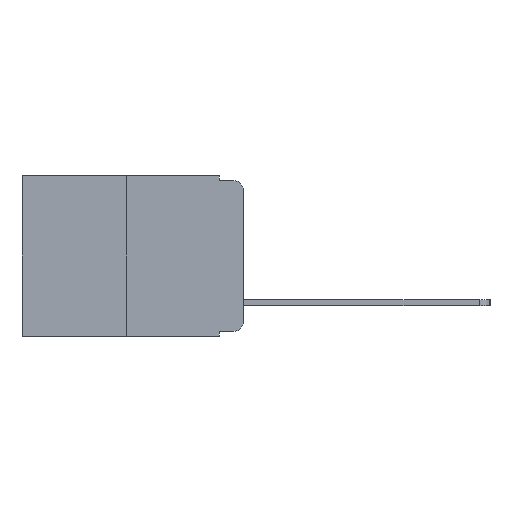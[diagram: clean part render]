
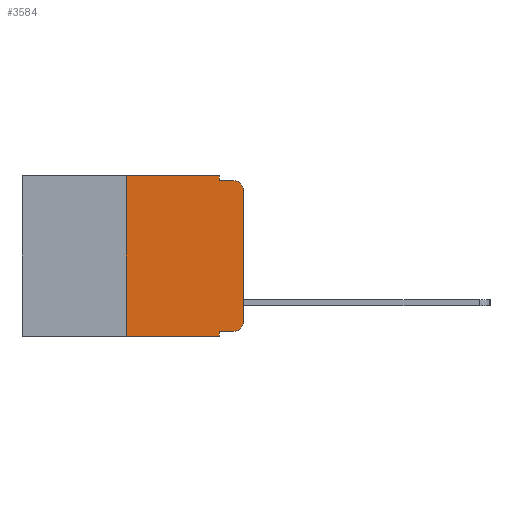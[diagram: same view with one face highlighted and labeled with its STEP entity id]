
A CAD part, left-side view. The second image highlights one B-rep face of the part: STEP entity #3584.
In plain terms, the highlighted planar face has unit normal (-1, 0, 0).
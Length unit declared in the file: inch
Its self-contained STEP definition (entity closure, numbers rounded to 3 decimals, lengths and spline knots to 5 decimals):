
#1 = CARTESIAN_POINT ( 'NONE',  ( 0., 0.25, -0.343 ) ) ;
#11 = EDGE_CURVE ( 'NONE', #4021, #7006, #10398, .T. ) ;
#295 = CARTESIAN_POINT ( 'NONE',  ( 0., 0., 0. ) ) ;
#320 = CARTESIAN_POINT ( 'NONE',  ( 0., 0.051, -0.333 ) ) ;
#432 = EDGE_CURVE ( 'NONE', #691, #3779, #3934, .T. ) ;
#502 = EDGE_CURVE ( 'NONE', #691, #6331, #7375, .T. ) ;
#691 = VERTEX_POINT ( 'NONE', #1 ) ;
#850 = VECTOR ( 'NONE', #9509, 39.37008 ) ;
#1102 = CARTESIAN_POINT ( 'NONE',  ( 0., 0.051, -0.333 ) ) ;
#1162 = VERTEX_POINT ( 'NONE', #320 ) ;
#1263 = CARTESIAN_POINT ( 'NONE',  ( 0., 0.051, -0.01 ) ) ;
#1444 = DIRECTION ( 'NONE',  ( -1., 0., 0. ) ) ;
#1470 = VECTOR ( 'NONE', #6472, 39.37008 ) ;
#1531 = VERTEX_POINT ( 'NONE', #2167 ) ;
#1986 = VECTOR ( 'NONE', #3161, 39.37008 ) ;
#2056 = VERTEX_POINT ( 'NONE', #5298 ) ;
#2109 = VECTOR ( 'NONE', #8835, 39.37008 ) ;
#2159 = LINE ( 'NONE', #10298, #4240 ) ;
#2167 = CARTESIAN_POINT ( 'NONE',  ( 0., 0.051, 0. ) ) ;
#2292 = CARTESIAN_POINT ( 'NONE',  ( 0., 0.25, 0. ) ) ;
#2390 = CARTESIAN_POINT ( 'NONE',  ( 0., 0.051, -0.343 ) ) ;
#2724 = VERTEX_POINT ( 'NONE', #9050 ) ;
#2893 = AXIS2_PLACEMENT_3D ( 'NONE', #6483, #7558, #7539 ) ;
#3161 = DIRECTION ( 'NONE',  ( 0., 0., -1. ) ) ;
#3313 = EDGE_CURVE ( 'NONE', #7006, #8983, #10348, .T. ) ;
#3584 = ADVANCED_FACE ( 'NONE', ( #10341 ), #9592, .F. ) ;
#3779 = VERTEX_POINT ( 'NONE', #2292 ) ;
#3827 = CARTESIAN_POINT ( 'NONE',  ( 0., 0., -0.03 ) ) ;
#3934 = LINE ( 'NONE', #7896, #1470 ) ;
#4021 = VERTEX_POINT ( 'NONE', #8584 ) ;
#4190 = EDGE_CURVE ( 'NONE', #3779, #1531, #2159, .T. ) ;
#4240 = VECTOR ( 'NONE', #8830, 39.37008 ) ;
#4347 = ORIENTED_EDGE ( 'NONE', *, *, #11, .T. ) ;
#4392 = ORIENTED_EDGE ( 'NONE', *, *, #9510, .T. ) ;
#4400 = ORIENTED_EDGE ( 'NONE', *, *, #3313, .T. ) ;
#4497 = EDGE_LOOP ( 'NONE', ( #4347, #4400, #4633, #4656, #8241, #7687, #6742, #6384, #4676, #4392 ) ) ;
#4633 = ORIENTED_EDGE ( 'NONE', *, *, #4934, .F. ) ;
#4656 = ORIENTED_EDGE ( 'NONE', *, *, #8006, .F. ) ;
#4676 = ORIENTED_EDGE ( 'NONE', *, *, #7090, .T. ) ;
#4934 = EDGE_CURVE ( 'NONE', #2724, #8983, #6687, .T. ) ;
#5298 = CARTESIAN_POINT ( 'NONE',  ( 0., 0.02, -0.333 ) ) ;
#5483 = VECTOR ( 'NONE', #9783, 39.37008 ) ;
#5706 = VECTOR ( 'NONE', #9941, 39.37008 ) ;
#5717 = LINE ( 'NONE', #7666, #5483 ) ;
#5943 = DIRECTION ( 'NONE',  ( 0., 0., -1. ) ) ;
#6331 = VERTEX_POINT ( 'NONE', #2390 ) ;
#6347 = CARTESIAN_POINT ( 'NONE',  ( 0., 0.051, 0. ) ) ;
#6384 = ORIENTED_EDGE ( 'NONE', *, *, #6588, .F. ) ;
#6385 = DIRECTION ( 'NONE',  ( -1., 0., 0. ) ) ;
#6472 = DIRECTION ( 'NONE',  ( 0., 0., 1. ) ) ;
#6483 = CARTESIAN_POINT ( 'NONE',  ( 0., 0.473, 0. ) ) ;
#6540 = CARTESIAN_POINT ( 'NONE',  ( 0., 0.02, -0.313 ) ) ;
#6588 = EDGE_CURVE ( 'NONE', #1162, #6331, #5717, .T. ) ;
#6687 = LINE ( 'NONE', #1263, #8615 ) ;
#6696 = LINE ( 'NONE', #6347, #1986 ) ;
#6742 = ORIENTED_EDGE ( 'NONE', *, *, #502, .T. ) ;
#7006 = VERTEX_POINT ( 'NONE', #3827 ) ;
#7090 = EDGE_CURVE ( 'NONE', #1162, #2056, #7758, .T. ) ;
#7177 = DIRECTION ( 'NONE',  ( 0., -1., 0. ) ) ;
#7323 = DIRECTION ( 'NONE',  ( 0., 0., -1. ) ) ;
#7375 = LINE ( 'NONE', #10289, #850 ) ;
#7397 = CIRCLE ( 'NONE', #7849, 0.02 ) ;
#7539 = DIRECTION ( 'NONE',  ( 0., 0., -1. ) ) ;
#7558 = DIRECTION ( 'NONE',  ( 1., 0., 0. ) ) ;
#7666 = CARTESIAN_POINT ( 'NONE',  ( 0., 0.051, 0. ) ) ;
#7687 = ORIENTED_EDGE ( 'NONE', *, *, #432, .F. ) ;
#7758 = LINE ( 'NONE', #1102, #5706 ) ;
#7849 = AXIS2_PLACEMENT_3D ( 'NONE', #6540, #1444, #7323 ) ;
#7896 = CARTESIAN_POINT ( 'NONE',  ( 0., 0.25, 0. ) ) ;
#8006 = EDGE_CURVE ( 'NONE', #1531, #2724, #6696, .T. ) ;
#8241 = ORIENTED_EDGE ( 'NONE', *, *, #4190, .F. ) ;
#8584 = CARTESIAN_POINT ( 'NONE',  ( 0., 0., -0.313 ) ) ;
#8615 = VECTOR ( 'NONE', #7177, 39.37008 ) ;
#8694 = AXIS2_PLACEMENT_3D ( 'NONE', #9850, #6385, #5943 ) ;
#8830 = DIRECTION ( 'NONE',  ( 0., -1., 0. ) ) ;
#8835 = DIRECTION ( 'NONE',  ( 0., 0., 1. ) ) ;
#8983 = VERTEX_POINT ( 'NONE', #9519 ) ;
#9050 = CARTESIAN_POINT ( 'NONE',  ( 0., 0.051, -0.01 ) ) ;
#9509 = DIRECTION ( 'NONE',  ( 0., -1., 0. ) ) ;
#9510 = EDGE_CURVE ( 'NONE', #2056, #4021, #7397, .T. ) ;
#9519 = CARTESIAN_POINT ( 'NONE',  ( 0., 0.02, -0.01 ) ) ;
#9592 = PLANE ( 'NONE',  #2893 ) ;
#9783 = DIRECTION ( 'NONE',  ( 0., 0., -1. ) ) ;
#9850 = CARTESIAN_POINT ( 'NONE',  ( 0., 0.02, -0.03 ) ) ;
#9941 = DIRECTION ( 'NONE',  ( 0., -1., 0. ) ) ;
#10289 = CARTESIAN_POINT ( 'NONE',  ( 0., 0.473, -0.343 ) ) ;
#10298 = CARTESIAN_POINT ( 'NONE',  ( 0., 0.473, 0. ) ) ;
#10341 = FACE_OUTER_BOUND ( 'NONE', #4497, .T. ) ;
#10348 = CIRCLE ( 'NONE', #8694, 0.02 ) ;
#10398 = LINE ( 'NONE', #295, #2109 ) ;
